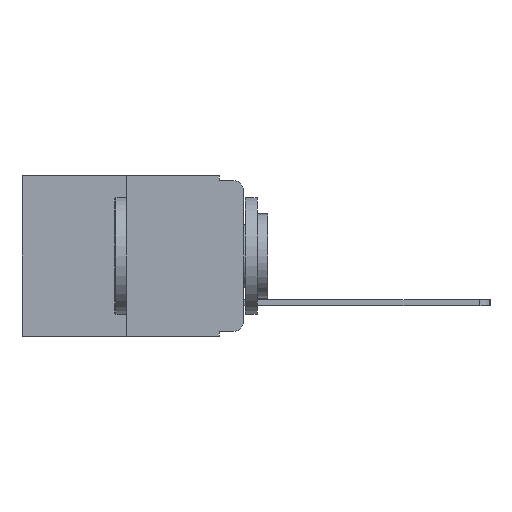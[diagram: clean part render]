
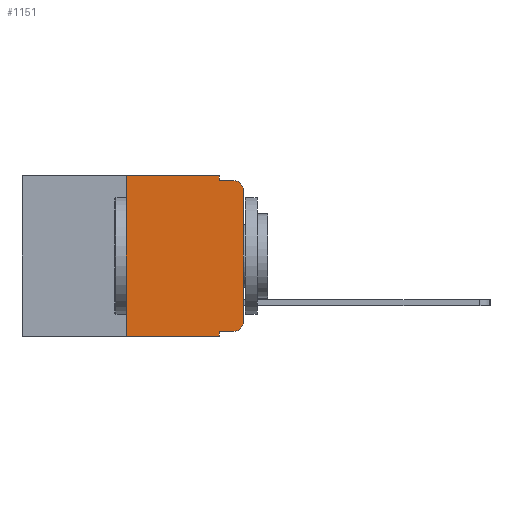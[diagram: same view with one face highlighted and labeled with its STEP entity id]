
A CAD part, left-side view. The second image highlights one B-rep face of the part: STEP entity #1151.
In plain terms, the highlighted planar face has unit normal (-1, 0, 0).
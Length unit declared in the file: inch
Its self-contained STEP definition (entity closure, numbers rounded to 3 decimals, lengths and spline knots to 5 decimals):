
#191 = VECTOR ( 'NONE', #7884, 39.37008 ) ;
#839 = ORIENTED_EDGE ( 'NONE', *, *, #17526, .F. ) ;
#894 = VECTOR ( 'NONE', #1660, 39.37008 ) ;
#1005 = CARTESIAN_POINT ( 'NONE',  ( 0., 0.051, -0.333 ) ) ;
#1058 = DIRECTION ( 'NONE',  ( 0., 0., -1. ) ) ;
#1151 = ADVANCED_FACE ( 'NONE', ( #1945 ), #4474, .F. ) ;
#1374 = LINE ( 'NONE', #13713, #15478 ) ;
#1595 = ORIENTED_EDGE ( 'NONE', *, *, #17220, .T. ) ;
#1660 = DIRECTION ( 'NONE',  ( 0., 0., 1. ) ) ;
#1772 = VERTEX_POINT ( 'NONE', #1005 ) ;
#1945 = FACE_OUTER_BOUND ( 'NONE', #12759, .T. ) ;
#1950 = VECTOR ( 'NONE', #6258, 39.37008 ) ;
#2445 = EDGE_CURVE ( 'NONE', #5015, #9982, #7040, .T. ) ;
#2774 = LINE ( 'NONE', #7941, #9799 ) ;
#2810 = CIRCLE ( 'NONE', #10139, 0.02 ) ;
#3650 = CARTESIAN_POINT ( 'NONE',  ( 0., 0.051, -0.01 ) ) ;
#3730 = CARTESIAN_POINT ( 'NONE',  ( 0., 0.051, 0. ) ) ;
#3983 = CARTESIAN_POINT ( 'NONE',  ( 0., 0.051, 0. ) ) ;
#4175 = CARTESIAN_POINT ( 'NONE',  ( 0., 0.473, -0.343 ) ) ;
#4318 = AXIS2_PLACEMENT_3D ( 'NONE', #17736, #4511, #4764 ) ;
#4474 = PLANE ( 'NONE',  #4318 ) ;
#4482 = CARTESIAN_POINT ( 'NONE',  ( 0., 0.02, -0.01 ) ) ;
#4511 = DIRECTION ( 'NONE',  ( 1., 0., 0. ) ) ;
#4699 = EDGE_CURVE ( 'NONE', #6438, #17426, #2774, .T. ) ;
#4764 = DIRECTION ( 'NONE',  ( 0., 0., -1. ) ) ;
#4778 = LINE ( 'NONE', #11881, #191 ) ;
#4913 = CARTESIAN_POINT ( 'NONE',  ( 0., 0.051, -0.333 ) ) ;
#5015 = VERTEX_POINT ( 'NONE', #5888 ) ;
#5126 = AXIS2_PLACEMENT_3D ( 'NONE', #14377, #6397, #15653 ) ;
#5269 = VERTEX_POINT ( 'NONE', #9040 ) ;
#5789 = CARTESIAN_POINT ( 'NONE',  ( 0., 0.051, -0.343 ) ) ;
#5888 = CARTESIAN_POINT ( 'NONE',  ( 0., 0.25, -0.343 ) ) ;
#6173 = LINE ( 'NONE', #4913, #1950 ) ;
#6224 = CARTESIAN_POINT ( 'NONE',  ( 0., 0.051, -0.01 ) ) ;
#6258 = DIRECTION ( 'NONE',  ( 0., -1., 0. ) ) ;
#6397 = DIRECTION ( 'NONE',  ( -1., 0., 0. ) ) ;
#6438 = VERTEX_POINT ( 'NONE', #9740 ) ;
#6504 = CIRCLE ( 'NONE', #5126, 0.02 ) ;
#6608 = LINE ( 'NONE', #3983, #16669 ) ;
#7040 = LINE ( 'NONE', #4175, #13690 ) ;
#7884 = DIRECTION ( 'NONE',  ( 0., 0., 1. ) ) ;
#7941 = CARTESIAN_POINT ( 'NONE',  ( 0., 0.473, 0. ) ) ;
#9040 = CARTESIAN_POINT ( 'NONE',  ( 0., 0.02, -0.333 ) ) ;
#9432 = ORIENTED_EDGE ( 'NONE', *, *, #14969, .T. ) ;
#9645 = ORIENTED_EDGE ( 'NONE', *, *, #15511, .T. ) ;
#9684 = DIRECTION ( 'NONE',  ( -1., 0., 0. ) ) ;
#9740 = CARTESIAN_POINT ( 'NONE',  ( 0., 0.25, 0. ) ) ;
#9799 = VECTOR ( 'NONE', #15755, 39.37008 ) ;
#9982 = VERTEX_POINT ( 'NONE', #5789 ) ;
#9983 = VERTEX_POINT ( 'NONE', #4482 ) ;
#10139 = AXIS2_PLACEMENT_3D ( 'NONE', #17333, #9684, #1058 ) ;
#10488 = ORIENTED_EDGE ( 'NONE', *, *, #12983, .F. ) ;
#10868 = LINE ( 'NONE', #6224, #11258 ) ;
#11105 = CARTESIAN_POINT ( 'NONE',  ( 0., 0., -0.03 ) ) ;
#11209 = DIRECTION ( 'NONE',  ( 0., 0., -1. ) ) ;
#11256 = EDGE_CURVE ( 'NONE', #5015, #6438, #4778, .T. ) ;
#11258 = VECTOR ( 'NONE', #16779, 39.37008 ) ;
#11881 = CARTESIAN_POINT ( 'NONE',  ( 0., 0.25, 0. ) ) ;
#12093 = ORIENTED_EDGE ( 'NONE', *, *, #16671, .T. ) ;
#12540 = VERTEX_POINT ( 'NONE', #3650 ) ;
#12759 = EDGE_LOOP ( 'NONE', ( #1595, #9645, #16436, #10488, #13861, #17246, #15048, #839, #12093, #9432 ) ) ;
#12983 = EDGE_CURVE ( 'NONE', #17426, #12540, #1374, .T. ) ;
#13690 = VECTOR ( 'NONE', #16676, 39.37008 ) ;
#13713 = CARTESIAN_POINT ( 'NONE',  ( 0., 0.051, 0. ) ) ;
#13861 = ORIENTED_EDGE ( 'NONE', *, *, #4699, .F. ) ;
#14377 = CARTESIAN_POINT ( 'NONE',  ( 0., 0.02, -0.03 ) ) ;
#14662 = EDGE_CURVE ( 'NONE', #12540, #9983, #10868, .T. ) ;
#14886 = CARTESIAN_POINT ( 'NONE',  ( 0., 0., -0.313 ) ) ;
#14969 = EDGE_CURVE ( 'NONE', #5269, #15023, #2810, .T. ) ;
#15023 = VERTEX_POINT ( 'NONE', #14886 ) ;
#15048 = ORIENTED_EDGE ( 'NONE', *, *, #2445, .T. ) ;
#15478 = VECTOR ( 'NONE', #11209, 39.37008 ) ;
#15496 = LINE ( 'NONE', #17782, #894 ) ;
#15511 = EDGE_CURVE ( 'NONE', #15868, #9983, #6504, .T. ) ;
#15653 = DIRECTION ( 'NONE',  ( 0., 0., -1. ) ) ;
#15755 = DIRECTION ( 'NONE',  ( 0., -1., 0. ) ) ;
#15868 = VERTEX_POINT ( 'NONE', #11105 ) ;
#16436 = ORIENTED_EDGE ( 'NONE', *, *, #14662, .F. ) ;
#16669 = VECTOR ( 'NONE', #17182, 39.37008 ) ;
#16671 = EDGE_CURVE ( 'NONE', #1772, #5269, #6173, .T. ) ;
#16676 = DIRECTION ( 'NONE',  ( 0., -1., 0. ) ) ;
#16779 = DIRECTION ( 'NONE',  ( 0., -1., 0. ) ) ;
#17182 = DIRECTION ( 'NONE',  ( 0., 0., -1. ) ) ;
#17220 = EDGE_CURVE ( 'NONE', #15023, #15868, #15496, .T. ) ;
#17246 = ORIENTED_EDGE ( 'NONE', *, *, #11256, .F. ) ;
#17333 = CARTESIAN_POINT ( 'NONE',  ( 0., 0.02, -0.313 ) ) ;
#17426 = VERTEX_POINT ( 'NONE', #3730 ) ;
#17526 = EDGE_CURVE ( 'NONE', #1772, #9982, #6608, .T. ) ;
#17736 = CARTESIAN_POINT ( 'NONE',  ( 0., 0.473, 0. ) ) ;
#17782 = CARTESIAN_POINT ( 'NONE',  ( 0., 0., 0. ) ) ;
